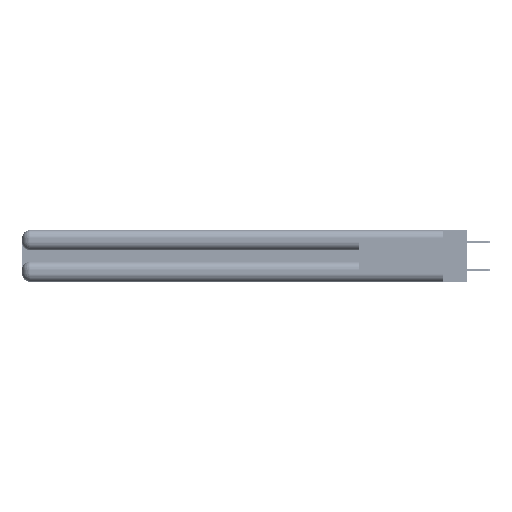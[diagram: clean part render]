
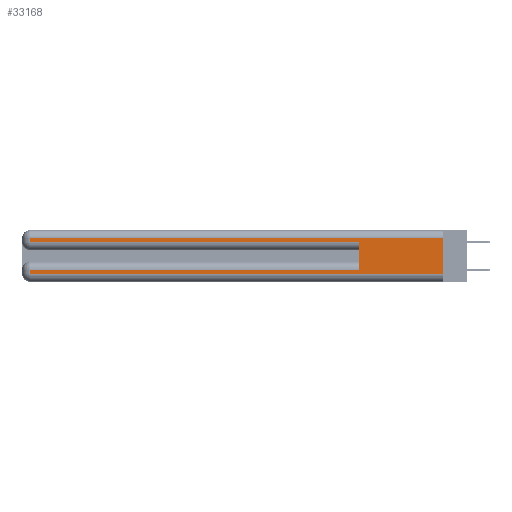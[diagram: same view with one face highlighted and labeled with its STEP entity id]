
A CAD part, left-side view. The second image highlights one B-rep face of the part: STEP entity #33168.
In plain terms, the highlighted planar face has unit normal (-1, 0, 0).
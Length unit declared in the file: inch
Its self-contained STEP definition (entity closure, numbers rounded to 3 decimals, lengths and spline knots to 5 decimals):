
#3419 = DIRECTION ( 'NONE',  ( 0., 0., -1. ) ) ;
#5617 = ORIENTED_EDGE ( 'NONE', *, *, #12178, .T. ) ;
#5754 = CARTESIAN_POINT ( 'NONE',  ( 0., 0., 0.06 ) ) ;
#5835 = EDGE_CURVE ( 'NONE', #26294, #45834, #53892, .T. ) ;
#6053 = CARTESIAN_POINT ( 'NONE',  ( 0., 0., 0.285 ) ) ;
#6631 = CARTESIAN_POINT ( 'NONE',  ( 0., 2.94, 0.31 ) ) ;
#10396 = DIRECTION ( 'NONE',  ( 0., -1., 0. ) ) ;
#10595 = ORIENTED_EDGE ( 'NONE', *, *, #30285, .T. ) ;
#11475 = VECTOR ( 'NONE', #52926, 39.37008 ) ;
#12178 = EDGE_CURVE ( 'NONE', #37515, #44280, #33192, .T. ) ;
#13972 = ORIENTED_EDGE ( 'NONE', *, *, #29713, .T. ) ;
#14206 = LINE ( 'NONE', #20920, #47198 ) ;
#15060 = LINE ( 'NONE', #55795, #22544 ) ;
#15248 = CARTESIAN_POINT ( 'NONE',  ( 0., 0.6, 0.085 ) ) ;
#18399 = VECTOR ( 'NONE', #20665, 39.37008 ) ;
#19565 = EDGE_CURVE ( 'NONE', #26294, #37515, #23695, .T. ) ;
#20665 = DIRECTION ( 'NONE',  ( 0., 0., -1. ) ) ;
#20727 = PLANE ( 'NONE',  #20794 ) ;
#20794 = AXIS2_PLACEMENT_3D ( 'NONE', #25085, #29415, #3419 ) ;
#20920 = CARTESIAN_POINT ( 'NONE',  ( 0., 0., 0.37 ) ) ;
#21034 = VECTOR ( 'NONE', #45434, 39.37008 ) ;
#22154 = ORIENTED_EDGE ( 'NONE', *, *, #19565, .T. ) ;
#22360 = VECTOR ( 'NONE', #40666, 39.37008 ) ;
#22544 = VECTOR ( 'NONE', #34545, 39.37008 ) ;
#23564 = CARTESIAN_POINT ( 'NONE',  ( 0., 0., 0.085 ) ) ;
#23695 = LINE ( 'NONE', #23564, #22360 ) ;
#24534 = CARTESIAN_POINT ( 'NONE',  ( 0., 0., 0.06 ) ) ;
#24551 = FACE_OUTER_BOUND ( 'NONE', #32060, .T. ) ;
#24919 = VERTEX_POINT ( 'NONE', #6631 ) ;
#25085 = CARTESIAN_POINT ( 'NONE',  ( 0., 0., 0.37 ) ) ;
#25257 = DIRECTION ( 'NONE',  ( 0., 0., -1. ) ) ;
#25420 = CARTESIAN_POINT ( 'NONE',  ( 0., 0.6, 0.285 ) ) ;
#25961 = CARTESIAN_POINT ( 'NONE',  ( 0., 2.94, 0.06 ) ) ;
#26186 = VERTEX_POINT ( 'NONE', #53026 ) ;
#26286 = CARTESIAN_POINT ( 'NONE',  ( 0., 2.94, 0.285 ) ) ;
#26294 = VERTEX_POINT ( 'NONE', #15248 ) ;
#27546 = DIRECTION ( 'NONE',  ( 0., -1., 0. ) ) ;
#27632 = CARTESIAN_POINT ( 'NONE',  ( 0., 2.94, 0.085 ) ) ;
#29415 = DIRECTION ( 'NONE',  ( 1., 0., 0. ) ) ;
#29713 = EDGE_CURVE ( 'NONE', #26186, #24919, #15060, .T. ) ;
#30285 = EDGE_CURVE ( 'NONE', #24919, #49128, #31272, .T. ) ;
#31022 = VECTOR ( 'NONE', #10396, 39.37008 ) ;
#31272 = LINE ( 'NONE', #42134, #18399 ) ;
#32060 = EDGE_LOOP ( 'NONE', ( #51035, #13972, #10595, #55071, #55662, #22154, #5617, #38150 ) ) ;
#33168 = ADVANCED_FACE ( 'NONE', ( #24551 ), #20727, .F. ) ;
#33192 = LINE ( 'NONE', #48652, #11475 ) ;
#34545 = DIRECTION ( 'NONE',  ( 0., 1., 0. ) ) ;
#37515 = VERTEX_POINT ( 'NONE', #27632 ) ;
#38150 = ORIENTED_EDGE ( 'NONE', *, *, #39005, .T. ) ;
#39005 = EDGE_CURVE ( 'NONE', #44280, #46984, #45715, .T. ) ;
#40666 = DIRECTION ( 'NONE',  ( 0., 1., 0. ) ) ;
#42134 = CARTESIAN_POINT ( 'NONE',  ( 0., 2.94, 0.37 ) ) ;
#44280 = VERTEX_POINT ( 'NONE', #25961 ) ;
#44416 = VECTOR ( 'NONE', #27546, 39.37008 ) ;
#45434 = DIRECTION ( 'NONE',  ( 0., 0., 1. ) ) ;
#45715 = LINE ( 'NONE', #5754, #44416 ) ;
#45834 = VERTEX_POINT ( 'NONE', #25420 ) ;
#46984 = VERTEX_POINT ( 'NONE', #24534 ) ;
#47198 = VECTOR ( 'NONE', #25257, 39.37008 ) ;
#48150 = EDGE_CURVE ( 'NONE', #49128, #45834, #53729, .T. ) ;
#48652 = CARTESIAN_POINT ( 'NONE',  ( 0., 2.94, 0.37 ) ) ;
#49128 = VERTEX_POINT ( 'NONE', #26286 ) ;
#49712 = CARTESIAN_POINT ( 'NONE',  ( 0., 0.6, 0.145 ) ) ;
#51035 = ORIENTED_EDGE ( 'NONE', *, *, #51996, .F. ) ;
#51996 = EDGE_CURVE ( 'NONE', #26186, #46984, #14206, .T. ) ;
#52926 = DIRECTION ( 'NONE',  ( 0., 0., -1. ) ) ;
#53026 = CARTESIAN_POINT ( 'NONE',  ( 0., 0., 0.31 ) ) ;
#53729 = LINE ( 'NONE', #6053, #31022 ) ;
#53892 = LINE ( 'NONE', #49712, #21034 ) ;
#55071 = ORIENTED_EDGE ( 'NONE', *, *, #48150, .T. ) ;
#55662 = ORIENTED_EDGE ( 'NONE', *, *, #5835, .F. ) ;
#55795 = CARTESIAN_POINT ( 'NONE',  ( 0., 0., 0.31 ) ) ;
